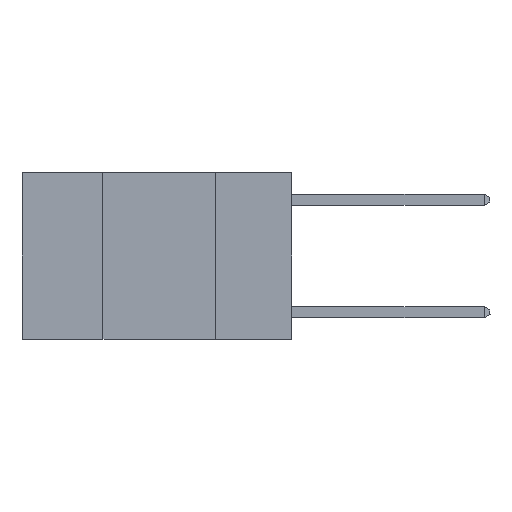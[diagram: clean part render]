
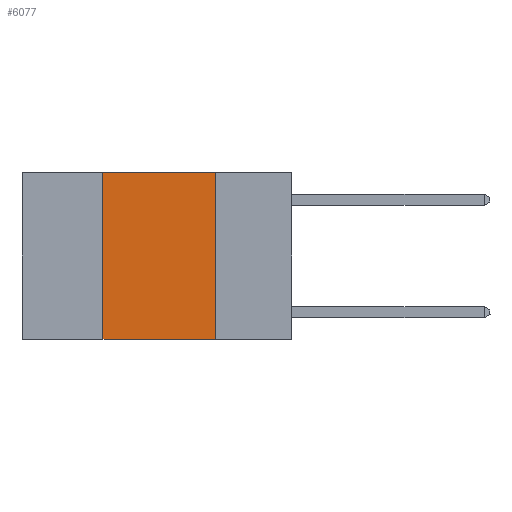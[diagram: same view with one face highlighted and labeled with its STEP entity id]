
A CAD part, left-side view. The second image highlights one B-rep face of the part: STEP entity #6077.
In plain terms, the highlighted planar face has unit normal (-1, 0, 0).
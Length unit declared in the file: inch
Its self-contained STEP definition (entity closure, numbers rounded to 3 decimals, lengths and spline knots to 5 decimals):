
#142 = VERTEX_POINT ( 'NONE', #18154 ) ;
#275 = PLANE ( 'NONE',  #18884 ) ;
#1670 = CARTESIAN_POINT ( 'NONE',  ( 0., 0.6, 0. ) ) ;
#2240 = DIRECTION ( 'NONE',  ( 0., 0., 1. ) ) ;
#3573 = DIRECTION ( 'NONE',  ( 0., -1., 0. ) ) ;
#3974 = DIRECTION ( 'NONE',  ( 0., 0., -1. ) ) ;
#4231 = LINE ( 'NONE', #20828, #8557 ) ;
#6077 = ADVANCED_FACE ( 'NONE', ( #17343 ), #275, .F. ) ;
#6835 = DIRECTION ( 'NONE',  ( 0., -1., 0. ) ) ;
#6838 = ORIENTED_EDGE ( 'NONE', *, *, #9959, .F. ) ;
#7240 = VERTEX_POINT ( 'NONE', #11957 ) ;
#7561 = VERTEX_POINT ( 'NONE', #14596 ) ;
#7938 = CARTESIAN_POINT ( 'NONE',  ( 0., 0.17, 0. ) ) ;
#8557 = VECTOR ( 'NONE', #6835, 39.37008 ) ;
#9959 = EDGE_CURVE ( 'NONE', #12666, #7240, #15259, .T. ) ;
#10120 = EDGE_CURVE ( 'NONE', #7561, #12666, #16653, .T. ) ;
#10289 = CARTESIAN_POINT ( 'NONE',  ( 0., 0.17, 0. ) ) ;
#11051 = ORIENTED_EDGE ( 'NONE', *, *, #10120, .F. ) ;
#11912 = VECTOR ( 'NONE', #3573, 39.37008 ) ;
#11957 = CARTESIAN_POINT ( 'NONE',  ( 0., 0.17, -0.37 ) ) ;
#12326 = ORIENTED_EDGE ( 'NONE', *, *, #20723, .F. ) ;
#12666 = VERTEX_POINT ( 'NONE', #7938 ) ;
#12894 = CARTESIAN_POINT ( 'NONE',  ( 0., 0.6, 0. ) ) ;
#14596 = CARTESIAN_POINT ( 'NONE',  ( 0., 0.42, 0. ) ) ;
#14723 = DIRECTION ( 'NONE',  ( 1., 0., 0. ) ) ;
#15259 = LINE ( 'NONE', #10289, #19354 ) ;
#16590 = ORIENTED_EDGE ( 'NONE', *, *, #22377, .T. ) ;
#16653 = LINE ( 'NONE', #1670, #11912 ) ;
#17153 = VECTOR ( 'NONE', #2240, 39.37008 ) ;
#17343 = FACE_OUTER_BOUND ( 'NONE', #18657, .T. ) ;
#18154 = CARTESIAN_POINT ( 'NONE',  ( 0., 0.42, -0.37 ) ) ;
#18367 = CARTESIAN_POINT ( 'NONE',  ( 0., 0.42, 0. ) ) ;
#18657 = EDGE_LOOP ( 'NONE', ( #6838, #11051, #12326, #16590 ) ) ;
#18884 = AXIS2_PLACEMENT_3D ( 'NONE', #12894, #14723, #3974 ) ;
#19354 = VECTOR ( 'NONE', #20820, 39.37008 ) ;
#20723 = EDGE_CURVE ( 'NONE', #142, #7561, #21620, .T. ) ;
#20820 = DIRECTION ( 'NONE',  ( 0., 0., -1. ) ) ;
#20828 = CARTESIAN_POINT ( 'NONE',  ( 0., 0.6, -0.37 ) ) ;
#21620 = LINE ( 'NONE', #18367, #17153 ) ;
#22377 = EDGE_CURVE ( 'NONE', #142, #7240, #4231, .T. ) ;
